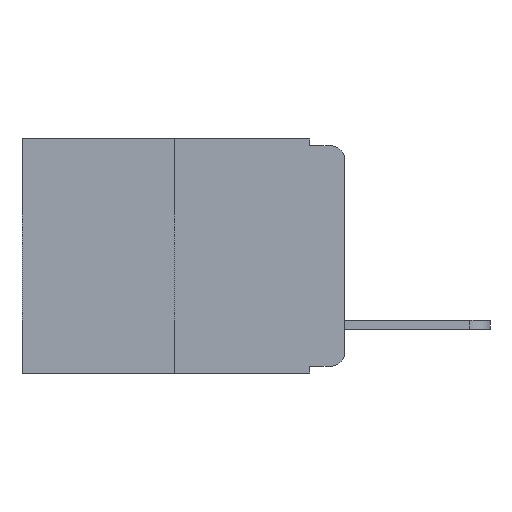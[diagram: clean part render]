
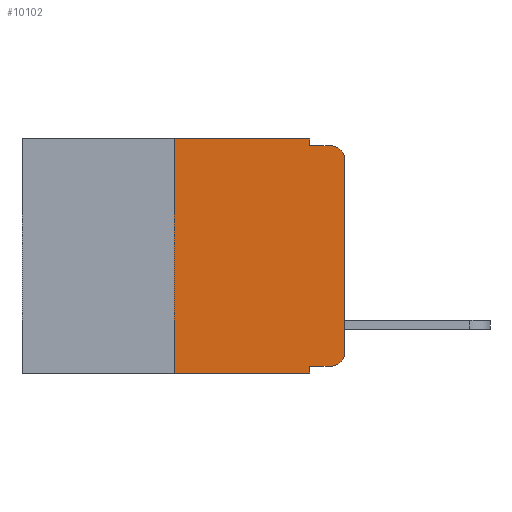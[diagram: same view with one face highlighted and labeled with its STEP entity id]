
A CAD part, left-side view. The second image highlights one B-rep face of the part: STEP entity #10102.
In plain terms, the highlighted planar face has unit normal (-1, 0, 0).
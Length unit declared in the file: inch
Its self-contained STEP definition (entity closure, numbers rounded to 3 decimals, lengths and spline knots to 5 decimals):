
#226 = CARTESIAN_POINT ( 'NONE',  ( 0., 0.051, -0.333 ) ) ;
#372 = DIRECTION ( 'NONE',  ( 0., -1., 0. ) ) ;
#409 = FACE_OUTER_BOUND ( 'NONE', #8492, .T. ) ;
#998 = LINE ( 'NONE', #11999, #8585 ) ;
#1463 = DIRECTION ( 'NONE',  ( -1., 0., 0. ) ) ;
#1479 = CARTESIAN_POINT ( 'NONE',  ( 0., 0.02, -0.313 ) ) ;
#1847 = VERTEX_POINT ( 'NONE', #10027 ) ;
#1879 = CARTESIAN_POINT ( 'NONE',  ( 0., 0.473, 0. ) ) ;
#2519 = VECTOR ( 'NONE', #11029, 39.37008 ) ;
#2599 = CARTESIAN_POINT ( 'NONE',  ( 0., 0.051, 0. ) ) ;
#2677 = LINE ( 'NONE', #5941, #9845 ) ;
#2723 = VERTEX_POINT ( 'NONE', #7164 ) ;
#3141 = CIRCLE ( 'NONE', #5497, 0.02 ) ;
#3210 = VECTOR ( 'NONE', #4382, 39.37008 ) ;
#3334 = VERTEX_POINT ( 'NONE', #5097 ) ;
#3352 = VECTOR ( 'NONE', #7538, 39.37008 ) ;
#3465 = CARTESIAN_POINT ( 'NONE',  ( 0., 0., 0. ) ) ;
#3671 = LINE ( 'NONE', #3983, #3352 ) ;
#3983 = CARTESIAN_POINT ( 'NONE',  ( 0., 0.051, -0.333 ) ) ;
#4231 = DIRECTION ( 'NONE',  ( 0., 0., -1. ) ) ;
#4242 = VERTEX_POINT ( 'NONE', #7977 ) ;
#4382 = DIRECTION ( 'NONE',  ( 0., -1., 0. ) ) ;
#4404 = CARTESIAN_POINT ( 'NONE',  ( 0., 0.02, -0.01 ) ) ;
#4490 = CARTESIAN_POINT ( 'NONE',  ( 0., 0.473, -0.343 ) ) ;
#4742 = VECTOR ( 'NONE', #11501, 39.37008 ) ;
#5097 = CARTESIAN_POINT ( 'NONE',  ( 0., 0.25, 0. ) ) ;
#5169 = CARTESIAN_POINT ( 'NONE',  ( 0., 0.051, -0.01 ) ) ;
#5333 = ORIENTED_EDGE ( 'NONE', *, *, #8474, .F. ) ;
#5383 = DIRECTION ( 'NONE',  ( 0., 0., -1. ) ) ;
#5407 = AXIS2_PLACEMENT_3D ( 'NONE', #1879, #8262, #5383 ) ;
#5441 = ORIENTED_EDGE ( 'NONE', *, *, #10609, .T. ) ;
#5463 = PLANE ( 'NONE',  #5407 ) ;
#5497 = AXIS2_PLACEMENT_3D ( 'NONE', #11802, #7278, #4231 ) ;
#5514 = DIRECTION ( 'NONE',  ( 0., 0., 1. ) ) ;
#5517 = EDGE_CURVE ( 'NONE', #3334, #5657, #998, .T. ) ;
#5657 = VERTEX_POINT ( 'NONE', #2599 ) ;
#5941 = CARTESIAN_POINT ( 'NONE',  ( 0., 0.25, 0. ) ) ;
#6335 = CARTESIAN_POINT ( 'NONE',  ( 0., 0.25, -0.343 ) ) ;
#6418 = LINE ( 'NONE', #11095, #11022 ) ;
#6623 = CARTESIAN_POINT ( 'NONE',  ( 0., 0., -0.313 ) ) ;
#6895 = EDGE_CURVE ( 'NONE', #8303, #8688, #8425, .T. ) ;
#7164 = CARTESIAN_POINT ( 'NONE',  ( 0., 0., -0.03 ) ) ;
#7180 = VERTEX_POINT ( 'NONE', #4404 ) ;
#7278 = DIRECTION ( 'NONE',  ( -1., 0., 0. ) ) ;
#7319 = LINE ( 'NONE', #10276, #4742 ) ;
#7538 = DIRECTION ( 'NONE',  ( 0., -1., 0. ) ) ;
#7698 = DIRECTION ( 'NONE',  ( 0., 0., -1. ) ) ;
#7866 = EDGE_CURVE ( 'NONE', #11834, #4242, #3671, .T. ) ;
#7977 = CARTESIAN_POINT ( 'NONE',  ( 0., 0.02, -0.333 ) ) ;
#8262 = DIRECTION ( 'NONE',  ( 1., 0., 0. ) ) ;
#8303 = VERTEX_POINT ( 'NONE', #6335 ) ;
#8404 = EDGE_CURVE ( 'NONE', #11834, #8688, #7319, .T. ) ;
#8425 = LINE ( 'NONE', #4490, #3210 ) ;
#8437 = EDGE_CURVE ( 'NONE', #4242, #10244, #11550, .T. ) ;
#8474 = EDGE_CURVE ( 'NONE', #5657, #1847, #6418, .T. ) ;
#8492 = EDGE_LOOP ( 'NONE', ( #5441, #8874, #9023, #5333, #9198, #9880, #9510, #10340, #10304, #10688 ) ) ;
#8533 = DIRECTION ( 'NONE',  ( 0., 0., 1. ) ) ;
#8543 = EDGE_CURVE ( 'NONE', #1847, #7180, #10253, .T. ) ;
#8585 = VECTOR ( 'NONE', #372, 39.37008 ) ;
#8688 = VERTEX_POINT ( 'NONE', #11105 ) ;
#8796 = EDGE_CURVE ( 'NONE', #8303, #3334, #2677, .T. ) ;
#8874 = ORIENTED_EDGE ( 'NONE', *, *, #9357, .T. ) ;
#8922 = VECTOR ( 'NONE', #8533, 39.37008 ) ;
#9023 = ORIENTED_EDGE ( 'NONE', *, *, #8543, .F. ) ;
#9198 = ORIENTED_EDGE ( 'NONE', *, *, #5517, .F. ) ;
#9210 = LINE ( 'NONE', #3465, #8922 ) ;
#9357 = EDGE_CURVE ( 'NONE', #2723, #7180, #3141, .T. ) ;
#9510 = ORIENTED_EDGE ( 'NONE', *, *, #6895, .T. ) ;
#9683 = AXIS2_PLACEMENT_3D ( 'NONE', #1479, #1463, #7698 ) ;
#9845 = VECTOR ( 'NONE', #5514, 39.37008 ) ;
#9880 = ORIENTED_EDGE ( 'NONE', *, *, #8796, .F. ) ;
#10027 = CARTESIAN_POINT ( 'NONE',  ( 0., 0.051, -0.01 ) ) ;
#10079 = DIRECTION ( 'NONE',  ( 0., 0., -1. ) ) ;
#10102 = ADVANCED_FACE ( 'NONE', ( #409 ), #5463, .F. ) ;
#10244 = VERTEX_POINT ( 'NONE', #6623 ) ;
#10253 = LINE ( 'NONE', #5169, #2519 ) ;
#10276 = CARTESIAN_POINT ( 'NONE',  ( 0., 0.051, 0. ) ) ;
#10304 = ORIENTED_EDGE ( 'NONE', *, *, #7866, .T. ) ;
#10340 = ORIENTED_EDGE ( 'NONE', *, *, #8404, .F. ) ;
#10609 = EDGE_CURVE ( 'NONE', #10244, #2723, #9210, .T. ) ;
#10688 = ORIENTED_EDGE ( 'NONE', *, *, #8437, .T. ) ;
#11022 = VECTOR ( 'NONE', #10079, 39.37008 ) ;
#11029 = DIRECTION ( 'NONE',  ( 0., -1., 0. ) ) ;
#11095 = CARTESIAN_POINT ( 'NONE',  ( 0., 0.051, 0. ) ) ;
#11105 = CARTESIAN_POINT ( 'NONE',  ( 0., 0.051, -0.343 ) ) ;
#11501 = DIRECTION ( 'NONE',  ( 0., 0., -1. ) ) ;
#11550 = CIRCLE ( 'NONE', #9683, 0.02 ) ;
#11802 = CARTESIAN_POINT ( 'NONE',  ( 0., 0.02, -0.03 ) ) ;
#11834 = VERTEX_POINT ( 'NONE', #226 ) ;
#11999 = CARTESIAN_POINT ( 'NONE',  ( 0., 0.473, 0. ) ) ;
